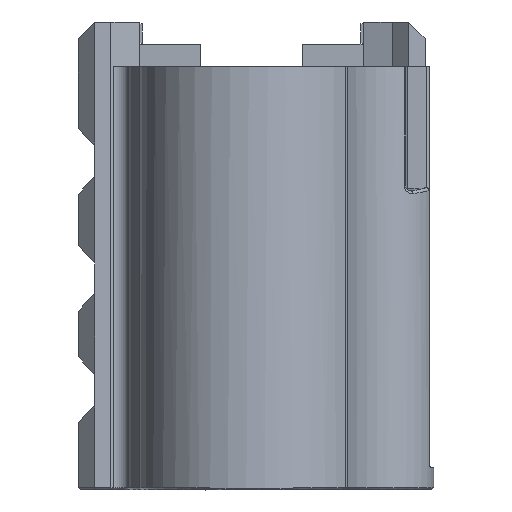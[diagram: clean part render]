
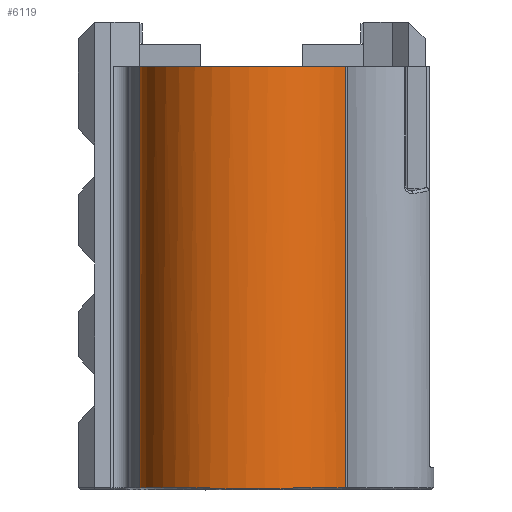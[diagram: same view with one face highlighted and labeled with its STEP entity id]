
A CAD part, front view. The second image highlights one B-rep face of the part: STEP entity #6119.
In plain terms, the highlighted cylindrical face has radius 20.1 mm (diameter 40.2 mm), a partial arc.
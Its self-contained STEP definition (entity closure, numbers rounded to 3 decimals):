
#27 = EDGE_CURVE ( 'NONE', #1878, #3769, #1463, .T. ) ;
#83 =( BOUNDED_CURVE ( )  B_SPLINE_CURVE ( 3, ( #7543, #2499, #1159, #5094 ),
 .UNSPECIFIED., .F., .T. ) 
 B_SPLINE_CURVE_WITH_KNOTS ( ( 4, 4 ),
 ( 4.549, 4.556 ),
 .UNSPECIFIED. ) 
 CURVE ( )  GEOMETRIC_REPRESENTATION_ITEM ( )  RATIONAL_B_SPLINE_CURVE ( ( 1., 1., 1., 1. ) ) 
 REPRESENTATION_ITEM ( '' )  );
#199 = CARTESIAN_POINT ( 'NONE',  ( 87.468, 67.412, 2.248 ) ) ;
#247 = CARTESIAN_POINT ( 'NONE',  ( 87.311, 58.32, -15.837 ) ) ;
#269 = CARTESIAN_POINT ( 'NONE',  ( 87.31, 57.916, 18.122 ) ) ;
#347 = B_SPLINE_CURVE_WITH_KNOTS ( 'NONE', 3,
 ( #4823, #6641, #7313, #2821, #3565, #7950, #4099, #960, #269, #6073, #2187, #2263, #3544, #2237, #2897, #5456, #7366, #1624, #6104, #6746, #4341, #7504 ),
 .UNSPECIFIED., .F., .F.,
 ( 4, 2, 2, 2, 2, 2, 2, 2, 2, 2, 4 ),
 ( 0., 0.003, 0.006, 0.009, 0.012, 0.013, 0.015, 0.018, 0.019, 0.02, 0.023 ),
 .UNSPECIFIED. ) ;
#460 = ORIENTED_EDGE ( 'NONE', *, *, #27, .T. ) ;
#523 = CARTESIAN_POINT ( 'NONE',  ( 87.312, 59.99, -14.655 ) ) ;
#600 = CARTESIAN_POINT ( 'NONE',  ( 87.318, 65.98, -6.524 ) ) ;
#700 = CYLINDRICAL_SURFACE ( 'NONE', #2900, 20.1 ) ;
#815 = DIRECTION ( 'NONE',  ( 0., 0., -1. ) ) ;
#867 = CARTESIAN_POINT ( 'NONE',  ( 87.465, 66.851, -3.999 ) ) ;
#906 = CARTESIAN_POINT ( 'NONE',  ( 87.7, 47.341, 1. ) ) ;
#933 = VERTEX_POINT ( 'NONE', #247 ) ;
#960 = CARTESIAN_POINT ( 'NONE',  ( 87.31, 57.075, 18.613 ) ) ;
#1137 = CARTESIAN_POINT ( 'NONE',  ( 87.316, 64.103, -10.141 ) ) ;
#1149 = VERTEX_POINT ( 'NONE', #5633 ) ;
#1159 = CARTESIAN_POINT ( 'NONE',  ( 87.414, 66.016, 8.434 ) ) ;
#1165 = DIRECTION ( 'NONE',  ( 0., 0., -1. ) ) ;
#1187 = CARTESIAN_POINT ( 'NONE',  ( 87.414, 66.016, -6.434 ) ) ;
#1220 = CARTESIAN_POINT ( 'NONE',  ( 87.315, 62.21, -12.565 ) ) ;
#1233 = LINE ( 'NONE', #4698, #4727 ) ;
#1463 = LINE ( 'NONE', #8148, #2158 ) ;
#1536 = CARTESIAN_POINT ( 'NONE',  ( 87.468, 67.412, -0.255 ) ) ;
#1590 = CARTESIAN_POINT ( 'NONE',  ( 87.467, 67.295, 3.498 ) ) ;
#1624 = CARTESIAN_POINT ( 'NONE',  ( 87.317, 64.165, 12.01 ) ) ;
#1729 = ORIENTED_EDGE ( 'NONE', *, *, #5951, .T. ) ;
#1878 = VERTEX_POINT ( 'NONE', #4440 ) ;
#2073 = B_SPLINE_CURVE_WITH_KNOTS ( 'NONE', 3,
 ( #4961, #3730, #4381, #1137, #3682, #1220, #5688, #523, #4990, #5608 ),
 .UNSPECIFIED., .F., .F.,
 ( 4, 2, 2, 2, 4 ),
 ( 0., 0.003, 0.006, 0.009, 0.012 ),
 .UNSPECIFIED. ) ;
#2158 = VECTOR ( 'NONE', #4287, 1000. ) ;
#2187 = CARTESIAN_POINT ( 'NONE',  ( 87.312, 59.524, 16.995 ) ) ;
#2237 = CARTESIAN_POINT ( 'NONE',  ( 87.314, 61.734, 15.064 ) ) ;
#2263 = CARTESIAN_POINT ( 'NONE',  ( 87.313, 60.292, 16.38 ) ) ;
#2360 = CIRCLE ( 'NONE', #5143, 20.1 ) ;
#2498 = CARTESIAN_POINT ( 'NONE',  ( 87.366, 65.998, -6.479 ) ) ;
#2499 = CARTESIAN_POINT ( 'NONE',  ( 87.366, 65.998, 8.479 ) ) ;
#2517 = VERTEX_POINT ( 'NONE', #5152 ) ;
#2645 = ORIENTED_EDGE ( 'NONE', *, *, #3772, .T. ) ;
#2749 = CARTESIAN_POINT ( 'NONE',  ( 87.464, 66.5, -5.209 ) ) ;
#2752 = VERTEX_POINT ( 'NONE', #3542 ) ;
#2779 = CARTESIAN_POINT ( 'NONE',  ( 87.462, 66.034, 8.389 ) ) ;
#2809 = CARTESIAN_POINT ( 'NONE',  ( 87.467, 67.294, -1.508 ) ) ;
#2821 = CARTESIAN_POINT ( 'NONE',  ( 87.304, 51.59, 20.67 ) ) ;
#2861 = CARTESIAN_POINT ( 'NONE',  ( 87.463, 66.267, 7.799 ) ) ;
#2897 = CARTESIAN_POINT ( 'NONE',  ( 87.315, 62.397, 14.352 ) ) ;
#2900 = AXIS2_PLACEMENT_3D ( 'NONE', #906, #7221, #815 ) ;
#3153 = EDGE_CURVE ( 'NONE', #933, #4380, #1233, .T. ) ;
#3178 = EDGE_CURVE ( 'NONE', #2752, #1149, #8158, .T. ) ;
#3471 = CARTESIAN_POINT ( 'NONE',  ( 87.467, 67.205, -2.138 ) ) ;
#3542 = CARTESIAN_POINT ( 'NONE',  ( 87.462, 66.034, 8.389 ) ) ;
#3544 = CARTESIAN_POINT ( 'NONE',  ( 87.313, 60.662, 16.06 ) ) ;
#3565 = CARTESIAN_POINT ( 'NONE',  ( 87.305, 52.542, 20.441 ) ) ;
#3590 = ORIENTED_EDGE ( 'NONE', *, *, #4910, .T. ) ;
#3682 = CARTESIAN_POINT ( 'NONE',  ( 87.316, 63.515, -10.978 ) ) ;
#3730 = CARTESIAN_POINT ( 'NONE',  ( 87.318, 65.595, -7.478 ) ) ;
#3769 = VERTEX_POINT ( 'NONE', #4351 ) ;
#3772 = EDGE_CURVE ( 'NONE', #5027, #933, #2073, .T. ) ;
#3781 = CARTESIAN_POINT ( 'NONE',  ( 87.318, 65.98, -6.524 ) ) ;
#4061 = ORIENTED_EDGE ( 'NONE', *, *, #3153, .T. ) ;
#4099 = CARTESIAN_POINT ( 'NONE',  ( 87.308, 55.328, 19.471 ) ) ;
#4287 = DIRECTION ( 'NONE',  ( 1., 0., 0. ) ) ;
#4334 = CARTESIAN_POINT ( 'NONE',  ( 11.678, 58.32, -15.837 ) ) ;
#4341 = CARTESIAN_POINT ( 'NONE',  ( 87.318, 65.611, 9.439 ) ) ;
#4351 = CARTESIAN_POINT ( 'NONE',  ( 87.3, 47.703, 21.097 ) ) ;
#4380 = VERTEX_POINT ( 'NONE', #4334 ) ;
#4381 = CARTESIAN_POINT ( 'NONE',  ( 87.318, 65.142, -8.391 ) ) ;
#4440 = CARTESIAN_POINT ( 'NONE',  ( 11.678, 47.703, 21.097 ) ) ;
#4698 = CARTESIAN_POINT ( 'NONE',  ( 87.7, 58.32, -15.837 ) ) ;
#4727 = VECTOR ( 'NONE', #5981, 1000. ) ;
#4794 = ORIENTED_EDGE ( 'NONE', *, *, #7751, .T. ) ;
#4823 = CARTESIAN_POINT ( 'NONE',  ( 87.3, 47.703, 21.097 ) ) ;
#4910 = EDGE_CURVE ( 'NONE', #2517, #2752, #83, .T. ) ;
#4961 = CARTESIAN_POINT ( 'NONE',  ( 87.318, 65.98, -6.524 ) ) ;
#4990 = CARTESIAN_POINT ( 'NONE',  ( 87.312, 59.181, -15.275 ) ) ;
#5017 = CARTESIAN_POINT ( 'NONE',  ( 87.462, 66.034, -6.389 ) ) ;
#5027 = VERTEX_POINT ( 'NONE', #3781 ) ;
#5084 = ORIENTED_EDGE ( 'NONE', *, *, #3178, .T. ) ;
#5094 = CARTESIAN_POINT ( 'NONE',  ( 87.462, 66.034, 8.389 ) ) ;
#5143 = AXIS2_PLACEMENT_3D ( 'NONE', #5551, #5636, #1165 ) ;
#5152 = CARTESIAN_POINT ( 'NONE',  ( 87.318, 65.98, 8.524 ) ) ;
#5306 =( BOUNDED_CURVE ( )  B_SPLINE_CURVE ( 3, ( #5017, #1187, #2498, #600 ),
 .UNSPECIFIED., .F., .T. ) 
 B_SPLINE_CURVE_WITH_KNOTS ( ( 4, 4 ),
 ( 1.727, 1.734 ),
 .UNSPECIFIED. ) 
 CURVE ( )  GEOMETRIC_REPRESENTATION_ITEM ( )  RATIONAL_B_SPLINE_CURVE ( ( 1., 1., 1., 1. ) ) 
 REPRESENTATION_ITEM ( '' )  );
#5308 = CARTESIAN_POINT ( 'NONE',  ( 87.468, 67.441, 1.623 ) ) ;
#5359 = CARTESIAN_POINT ( 'NONE',  ( 87.467, 67.207, 4.124 ) ) ;
#5456 = CARTESIAN_POINT ( 'NONE',  ( 87.316, 63.314, 13.212 ) ) ;
#5503 = ORIENTED_EDGE ( 'NONE', *, *, #7357, .T. ) ;
#5551 = CARTESIAN_POINT ( 'NONE',  ( 11.678, 47.341, 1. ) ) ;
#5608 = CARTESIAN_POINT ( 'NONE',  ( 87.311, 58.32, -15.837 ) ) ;
#5633 = CARTESIAN_POINT ( 'NONE',  ( 87.462, 66.034, -6.389 ) ) ;
#5636 = DIRECTION ( 'NONE',  ( 1., 0., 0. ) ) ;
#5688 = CARTESIAN_POINT ( 'NONE',  ( 87.314, 61.504, -13.299 ) ) ;
#5951 = EDGE_CURVE ( 'NONE', #1149, #5027, #5306, .T. ) ;
#5981 = DIRECTION ( 'NONE',  ( -1., 0., 0. ) ) ;
#6039 = CARTESIAN_POINT ( 'NONE',  ( 87.468, 67.441, 0.371 ) ) ;
#6073 = CARTESIAN_POINT ( 'NONE',  ( 87.312, 59.127, 17.289 ) ) ;
#6104 = CARTESIAN_POINT ( 'NONE',  ( 87.317, 64.431, 11.593 ) ) ;
#6119 = ADVANCED_FACE ( 'NONE', ( #6801 ), #700, .T. ) ;
#6574 = CARTESIAN_POINT ( 'NONE',  ( 87.464, 66.472, 7.198 ) ) ;
#6641 = CARTESIAN_POINT ( 'NONE',  ( 87.301, 48.69, 21.079 ) ) ;
#6656 = CARTESIAN_POINT ( 'NONE',  ( 87.465, 66.824, 5.984 ) ) ;
#6746 = CARTESIAN_POINT ( 'NONE',  ( 87.318, 65.177, 10.321 ) ) ;
#6801 = FACE_OUTER_BOUND ( 'NONE', #6876, .T. ) ;
#6876 = EDGE_LOOP ( 'NONE', ( #5084, #1729, #2645, #4061, #5503, #460, #4794, #3590 ) ) ;
#7221 = DIRECTION ( 'NONE',  ( 1., 0., 0. ) ) ;
#7313 = CARTESIAN_POINT ( 'NONE',  ( 87.302, 49.664, 20.989 ) ) ;
#7331 = CARTESIAN_POINT ( 'NONE',  ( 87.462, 66.034, -6.389 ) ) ;
#7357 = EDGE_CURVE ( 'NONE', #4380, #1878, #2360, .T. ) ;
#7366 = CARTESIAN_POINT ( 'NONE',  ( 87.316, 63.607, 12.819 ) ) ;
#7504 = CARTESIAN_POINT ( 'NONE',  ( 87.318, 65.98, 8.524 ) ) ;
#7543 = CARTESIAN_POINT ( 'NONE',  ( 87.318, 65.98, 8.524 ) ) ;
#7751 = EDGE_CURVE ( 'NONE', #3769, #2517, #347, .T. ) ;
#7950 = CARTESIAN_POINT ( 'NONE',  ( 87.307, 54.42, 19.838 ) ) ;
#7960 = CARTESIAN_POINT ( 'NONE',  ( 87.466, 66.971, 5.369 ) ) ;
#8148 = CARTESIAN_POINT ( 'NONE',  ( 87.7, 47.703, 21.097 ) ) ;
#8158 = B_SPLINE_CURVE_WITH_KNOTS ( 'NONE', 3,
 ( #2779, #2861, #6574, #6656, #7960, #5359, #1590, #199, #5308, #6039, #1536, #2809, #3471, #867, #2749, #7331 ),
 .UNSPECIFIED., .F., .F.,
 ( 4, 2, 2, 2, 2, 2, 2, 4 ),
 ( 0., 0.002, 0.004, 0.006, 0.008, 0.01, 0.011, 0.015 ),
 .UNSPECIFIED. ) ;
